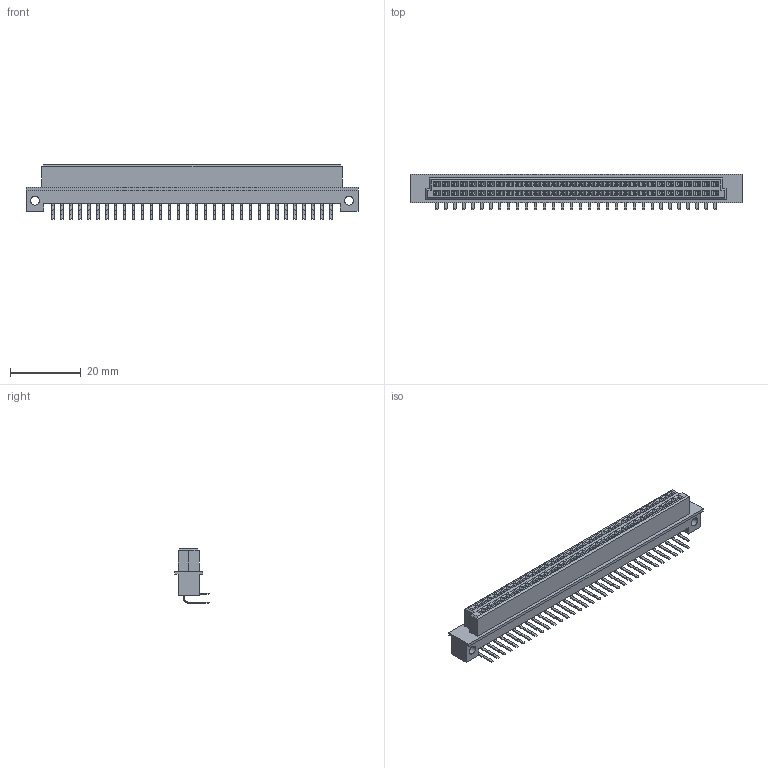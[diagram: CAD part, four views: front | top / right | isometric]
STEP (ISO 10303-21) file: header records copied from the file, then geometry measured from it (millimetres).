
FILE_DESCRIPTION (( 'STEP AP203' ), '1' );
FILE_NAME ('462-064-660-212.STEP', '2019-11-11T15:28:09', ( '' ), ( '' ), 'SwSTEP 2.0', 'SolidWorks 2020', '' );
FILE_SCHEMA (( 'CONFIG_CONTROL_DESIGN' ));
Length unit declared in the file: millimetre
Products named in the file (4): 462-290-1; 462 Part_64; 462-290-2; 462-064-660-212
Assembly tree (65 placements, depth 2):
  462-064-660-212
    462 Part_64
    462-290-1  x32
    462-290-2  x32
Bounding box: 94 x 9.9 x 15.43 mm (x, y, z)
Volume: 5650.3 mm3; surface area: 7447.1 mm2
Topology: 65 solids, 65 shells, 1763 faces, 4184 edges, 2616 vertices
Faces by surface type: plane 1631, cylinder 132
Entity records: 28136 total; most frequent: CARTESIAN_POINT 4539, ORIENTED_EDGE 4400, DIRECTION 4142, EDGE_CURVE 2200, VECTOR 2184, LINE 2184, VERTEX_POINT 1376, EDGE_LOOP 1092
